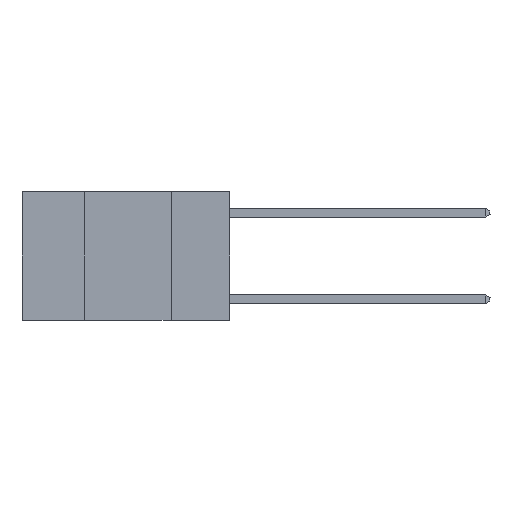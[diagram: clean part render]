
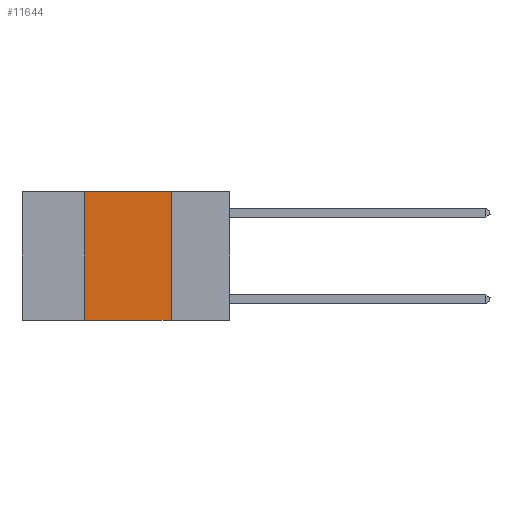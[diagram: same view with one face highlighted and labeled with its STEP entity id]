
A CAD part, left-side view. The second image highlights one B-rep face of the part: STEP entity #11644.
In plain terms, the highlighted planar face has unit normal (-1, 0, 0).
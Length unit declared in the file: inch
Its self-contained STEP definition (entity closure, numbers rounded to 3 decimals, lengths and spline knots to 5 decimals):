
#319 = LINE ( 'NONE', #7846, #14119 ) ;
#901 = CARTESIAN_POINT ( 'NONE',  ( 0., 0.42, 0. ) ) ;
#1464 = VECTOR ( 'NONE', #1781, 39.37008 ) ;
#1499 = LINE ( 'NONE', #8783, #6902 ) ;
#1781 = DIRECTION ( 'NONE',  ( 0., -1., 0. ) ) ;
#2149 = ORIENTED_EDGE ( 'NONE', *, *, #19255, .F. ) ;
#3654 = EDGE_CURVE ( 'NONE', #20619, #22724, #4625, .T. ) ;
#3793 = CARTESIAN_POINT ( 'NONE',  ( 0., 0.17, 0. ) ) ;
#4625 = LINE ( 'NONE', #901, #10597 ) ;
#6709 = DIRECTION ( 'NONE',  ( 0., 0., -1. ) ) ;
#6902 = VECTOR ( 'NONE', #14717, 39.37008 ) ;
#7560 = EDGE_LOOP ( 'NONE', ( #2149, #23511, #12362, #22081 ) ) ;
#7846 = CARTESIAN_POINT ( 'NONE',  ( 0., 0.17, 0. ) ) ;
#8783 = CARTESIAN_POINT ( 'NONE',  ( 0., 0.6, 0. ) ) ;
#9165 = PLANE ( 'NONE',  #14321 ) ;
#10597 = VECTOR ( 'NONE', #12157, 39.37008 ) ;
#11177 = LINE ( 'NONE', #18691, #1464 ) ;
#11644 = ADVANCED_FACE ( 'NONE', ( #12884 ), #9165, .F. ) ;
#12157 = DIRECTION ( 'NONE',  ( 0., 0., 1. ) ) ;
#12362 = ORIENTED_EDGE ( 'NONE', *, *, #3654, .F. ) ;
#12545 = CARTESIAN_POINT ( 'NONE',  ( 0., 0.42, -0.37 ) ) ;
#12884 = FACE_OUTER_BOUND ( 'NONE', #7560, .T. ) ;
#14119 = VECTOR ( 'NONE', #6709, 39.37008 ) ;
#14321 = AXIS2_PLACEMENT_3D ( 'NONE', #20528, #22490, #22980 ) ;
#14717 = DIRECTION ( 'NONE',  ( 0., -1., 0. ) ) ;
#16093 = VERTEX_POINT ( 'NONE', #3793 ) ;
#16822 = EDGE_CURVE ( 'NONE', #22724, #16093, #1499, .T. ) ;
#18691 = CARTESIAN_POINT ( 'NONE',  ( 0., 0.6, -0.37 ) ) ;
#18920 = CARTESIAN_POINT ( 'NONE',  ( 0., 0.17, -0.37 ) ) ;
#18973 = EDGE_CURVE ( 'NONE', #20619, #24369, #11177, .T. ) ;
#19255 = EDGE_CURVE ( 'NONE', #16093, #24369, #319, .T. ) ;
#20528 = CARTESIAN_POINT ( 'NONE',  ( 0., 0.6, 0. ) ) ;
#20619 = VERTEX_POINT ( 'NONE', #12545 ) ;
#21735 = CARTESIAN_POINT ( 'NONE',  ( 0., 0.42, 0. ) ) ;
#22081 = ORIENTED_EDGE ( 'NONE', *, *, #18973, .T. ) ;
#22490 = DIRECTION ( 'NONE',  ( 1., 0., 0. ) ) ;
#22724 = VERTEX_POINT ( 'NONE', #21735 ) ;
#22980 = DIRECTION ( 'NONE',  ( 0., 0., -1. ) ) ;
#23511 = ORIENTED_EDGE ( 'NONE', *, *, #16822, .F. ) ;
#24369 = VERTEX_POINT ( 'NONE', #18920 ) ;
